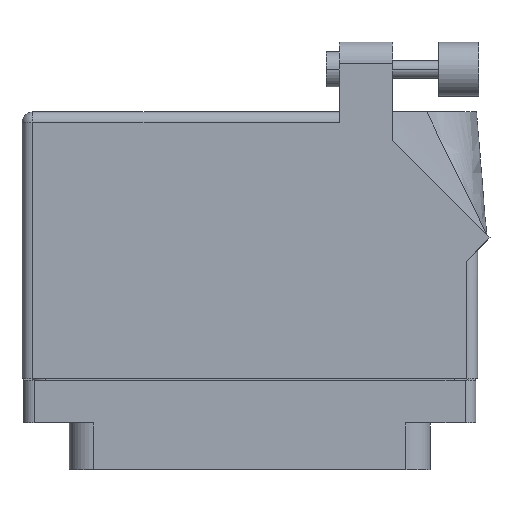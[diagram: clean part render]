
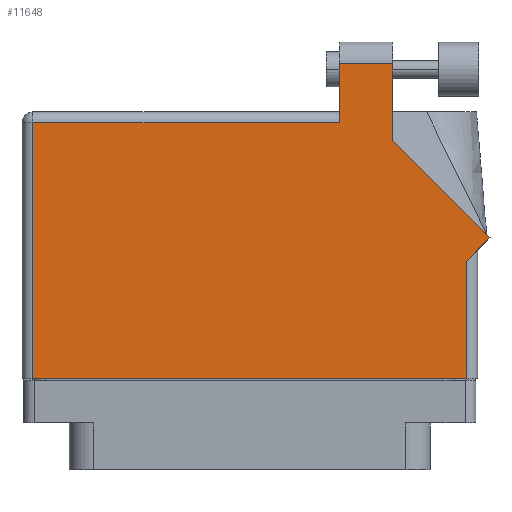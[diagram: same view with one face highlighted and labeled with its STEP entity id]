
A CAD part, front view. The second image highlights one B-rep face of the part: STEP entity #11648.
In plain terms, the highlighted face is planar.
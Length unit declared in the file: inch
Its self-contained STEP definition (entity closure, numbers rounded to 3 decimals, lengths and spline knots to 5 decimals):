
#2241 = EDGE_LOOP ( 'NONE', ( #13608, #8133, #26003, #39836, #26142, #43534, #31446, #27860, #12721 ) ) ;
#2597 = LINE ( 'NONE', #20331, #43179 ) ;
#4397 = DIRECTION ( 'NONE',  ( -1., 0., 0. ) ) ;
#5061 = EDGE_CURVE ( 'NONE', #26138, #12183, #16935, .T. ) ;
#7677 = CARTESIAN_POINT ( 'NONE',  ( 0.513, 1.368, 0.455 ) ) ;
#8133 = ORIENTED_EDGE ( 'NONE', *, *, #23456, .T. ) ;
#8534 = EDGE_CURVE ( 'NONE', #29004, #45974, #19439, .T. ) ;
#9011 = VECTOR ( 'NONE', #23824, 39.37008 ) ;
#9250 = CARTESIAN_POINT ( 'NONE',  ( 1.244, -0.1, 0.455 ) ) ;
#9253 = VECTOR ( 'NONE', #43877, 39.37008 ) ;
#9830 = LINE ( 'NONE', #25741, #9253 ) ;
#10024 = VECTOR ( 'NONE', #13173, 39.37008 ) ;
#10034 = EDGE_CURVE ( 'NONE', #41653, #26138, #9830, .T. ) ;
#10217 = VECTOR ( 'NONE', #21599, 39.37008 ) ;
#11041 = AXIS2_PLACEMENT_3D ( 'NONE', #19133, #44829, #34975 ) ;
#11648 = ADVANCED_FACE ( 'NONE', ( #42004 ), #37573, .F. ) ;
#12183 = VERTEX_POINT ( 'NONE', #43978 ) ;
#12721 = ORIENTED_EDGE ( 'NONE', *, *, #29388, .T. ) ;
#13173 = DIRECTION ( 'NONE',  ( 0., 1., 0. ) ) ;
#13608 = ORIENTED_EDGE ( 'NONE', *, *, #8534, .T. ) ;
#14139 = CARTESIAN_POINT ( 'NONE',  ( 1.306, 0.637, 0.455 ) ) ;
#14351 = CARTESIAN_POINT ( 'NONE',  ( -1.306, 1.368, 0.455 ) ) ;
#14383 = LINE ( 'NONE', #14351, #35231 ) ;
#15850 = VECTOR ( 'NONE', #35995, 39.37008 ) ;
#16935 = LINE ( 'NONE', #31656, #10024 ) ;
#17260 = VERTEX_POINT ( 'NONE', #24743 ) ;
#17733 = LINE ( 'NONE', #14139, #10217 ) ;
#19133 = CARTESIAN_POINT ( 'NONE',  ( -1.306, 1.43, 0.455 ) ) ;
#19356 = EDGE_CURVE ( 'NONE', #24552, #43662, #14383, .T. ) ;
#19439 = LINE ( 'NONE', #41899, #42595 ) ;
#19860 = VECTOR ( 'NONE', #4397, 39.37008 ) ;
#19953 = CARTESIAN_POINT ( 'NONE',  ( 0.513, 1.43, 0.455 ) ) ;
#20164 = DIRECTION ( 'NONE',  ( -0.707, 0.707, 0. ) ) ;
#20331 = CARTESIAN_POINT ( 'NONE',  ( 1.37671, 0.70771, 0.455 ) ) ;
#21599 = DIRECTION ( 'NONE',  ( 0.707, 0.707, 0. ) ) ;
#22972 = DIRECTION ( 'NONE',  ( 0., 1., 0. ) ) ;
#23456 = EDGE_CURVE ( 'NONE', #45974, #17260, #34917, .T. ) ;
#23824 = DIRECTION ( 'NONE',  ( 0., -1., 0. ) ) ;
#23883 = CARTESIAN_POINT ( 'NONE',  ( -1.244, 1.368, 0.455 ) ) ;
#24552 = VERTEX_POINT ( 'NONE', #7677 ) ;
#24743 = CARTESIAN_POINT ( 'NONE',  ( 0.513, 1.705, 0.455 ) ) ;
#24984 = VERTEX_POINT ( 'NONE', #38481 ) ;
#25213 = CARTESIAN_POINT ( 'NONE',  ( 0.82, 1.26442, 0.455 ) ) ;
#25741 = CARTESIAN_POINT ( 'NONE',  ( -1.306, -0.1, 0.455 ) ) ;
#26003 = ORIENTED_EDGE ( 'NONE', *, *, #35455, .T. ) ;
#26138 = VERTEX_POINT ( 'NONE', #9250 ) ;
#26142 = ORIENTED_EDGE ( 'NONE', *, *, #27285, .T. ) ;
#27285 = EDGE_CURVE ( 'NONE', #43662, #41653, #35559, .T. ) ;
#27860 = ORIENTED_EDGE ( 'NONE', *, *, #38491, .T. ) ;
#28542 = CARTESIAN_POINT ( 'NONE',  ( -1.244, -0.1, 0.455 ) ) ;
#29004 = VERTEX_POINT ( 'NONE', #25213 ) ;
#29388 = EDGE_CURVE ( 'NONE', #24984, #29004, #2597, .T. ) ;
#30236 = CARTESIAN_POINT ( 'NONE',  ( 0.513, 1.705, 0.455 ) ) ;
#31446 = ORIENTED_EDGE ( 'NONE', *, *, #5061, .T. ) ;
#31656 = CARTESIAN_POINT ( 'NONE',  ( 1.244, 0.637, 0.455 ) ) ;
#34917 = LINE ( 'NONE', #30236, #19860 ) ;
#34975 = DIRECTION ( 'NONE',  ( -1., 0., 0. ) ) ;
#35231 = VECTOR ( 'NONE', #47665, 39.37008 ) ;
#35455 = EDGE_CURVE ( 'NONE', #17260, #24552, #44335, .T. ) ;
#35559 = LINE ( 'NONE', #28542, #15850 ) ;
#35995 = DIRECTION ( 'NONE',  ( 0., -1., 0. ) ) ;
#37573 = PLANE ( 'NONE',  #11041 ) ;
#37744 = CARTESIAN_POINT ( 'NONE',  ( -1.244, -0.1, 0.455 ) ) ;
#38481 = CARTESIAN_POINT ( 'NONE',  ( 1.37671, 0.70771, 0.455 ) ) ;
#38491 = EDGE_CURVE ( 'NONE', #12183, #24984, #17733, .T. ) ;
#39836 = ORIENTED_EDGE ( 'NONE', *, *, #19356, .T. ) ;
#41653 = VERTEX_POINT ( 'NONE', #37744 ) ;
#41899 = CARTESIAN_POINT ( 'NONE',  ( 0.82, 1.26442, 0.455 ) ) ;
#42004 = FACE_OUTER_BOUND ( 'NONE', #2241, .T. ) ;
#42595 = VECTOR ( 'NONE', #22972, 39.37008 ) ;
#43179 = VECTOR ( 'NONE', #20164, 39.37008 ) ;
#43457 = CARTESIAN_POINT ( 'NONE',  ( 0.82, 1.705, 0.455 ) ) ;
#43534 = ORIENTED_EDGE ( 'NONE', *, *, #10034, .T. ) ;
#43662 = VERTEX_POINT ( 'NONE', #23883 ) ;
#43877 = DIRECTION ( 'NONE',  ( 1., 0., 0. ) ) ;
#43978 = CARTESIAN_POINT ( 'NONE',  ( 1.244, 0.575, 0.455 ) ) ;
#44335 = LINE ( 'NONE', #19953, #9011 ) ;
#44829 = DIRECTION ( 'NONE',  ( 0., 0., -1. ) ) ;
#45974 = VERTEX_POINT ( 'NONE', #43457 ) ;
#47665 = DIRECTION ( 'NONE',  ( -1., 0., 0. ) ) ;
